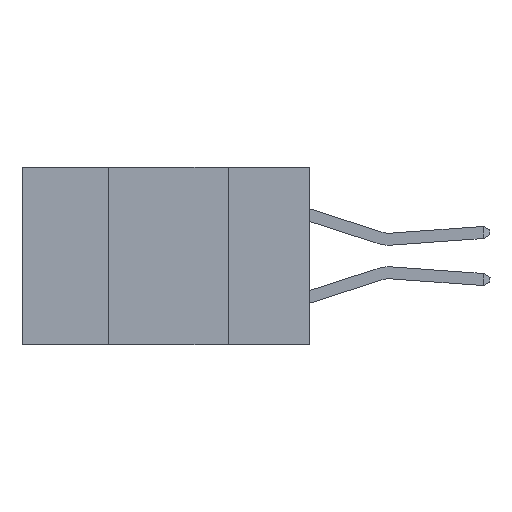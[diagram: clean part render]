
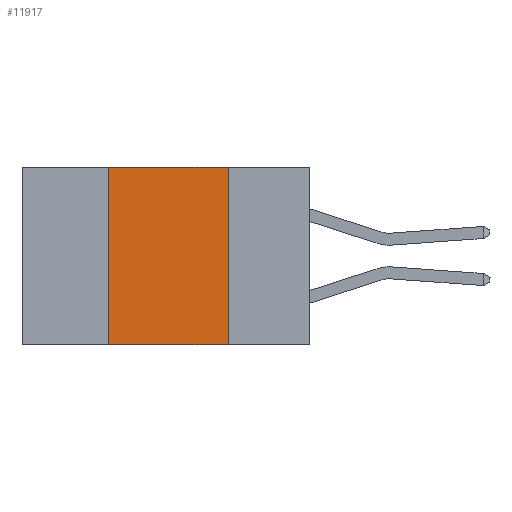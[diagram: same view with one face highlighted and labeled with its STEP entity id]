
A CAD part, left-side view. The second image highlights one B-rep face of the part: STEP entity #11917.
In plain terms, the highlighted planar face has unit normal (-1, 0, 0).
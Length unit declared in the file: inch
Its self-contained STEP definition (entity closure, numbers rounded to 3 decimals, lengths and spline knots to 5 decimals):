
#153 = FACE_OUTER_BOUND ( 'NONE', #10729, .T. ) ;
#1185 = ORIENTED_EDGE ( 'NONE', *, *, #19954, .F. ) ;
#1909 = DIRECTION ( 'NONE',  ( 1., 0., 0. ) ) ;
#2059 = VECTOR ( 'NONE', #17074, 39.37008 ) ;
#2104 = VERTEX_POINT ( 'NONE', #7624 ) ;
#2248 = CARTESIAN_POINT ( 'NONE',  ( 0., 0.17, -0.37 ) ) ;
#2817 = CARTESIAN_POINT ( 'NONE',  ( 0., 0.42, 0. ) ) ;
#3074 = LINE ( 'NONE', #8497, #19302 ) ;
#3381 = DIRECTION ( 'NONE',  ( 0., -1., 0. ) ) ;
#4059 = VERTEX_POINT ( 'NONE', #2248 ) ;
#5503 = ORIENTED_EDGE ( 'NONE', *, *, #12636, .F. ) ;
#6038 = DIRECTION ( 'NONE',  ( 0., 0., -1. ) ) ;
#6523 = LINE ( 'NONE', #17033, #9708 ) ;
#6775 = VECTOR ( 'NONE', #6038, 39.37008 ) ;
#7624 = CARTESIAN_POINT ( 'NONE',  ( 0., 0.42, 0. ) ) ;
#7852 = EDGE_CURVE ( 'NONE', #13060, #2104, #19563, .T. ) ;
#8497 = CARTESIAN_POINT ( 'NONE',  ( 0., 0.6, -0.37 ) ) ;
#8956 = ORIENTED_EDGE ( 'NONE', *, *, #7852, .F. ) ;
#9198 = DIRECTION ( 'NONE',  ( 0., -1., 0. ) ) ;
#9708 = VECTOR ( 'NONE', #9198, 39.37008 ) ;
#10729 = EDGE_LOOP ( 'NONE', ( #1185, #5503, #8956, #10933 ) ) ;
#10933 = ORIENTED_EDGE ( 'NONE', *, *, #15348, .T. ) ;
#11465 = PLANE ( 'NONE',  #15675 ) ;
#11917 = ADVANCED_FACE ( 'NONE', ( #153 ), #11465, .F. ) ;
#12118 = VERTEX_POINT ( 'NONE', #16066 ) ;
#12636 = EDGE_CURVE ( 'NONE', #2104, #12118, #6523, .T. ) ;
#12656 = CARTESIAN_POINT ( 'NONE',  ( 0., 0.42, -0.37 ) ) ;
#13060 = VERTEX_POINT ( 'NONE', #12656 ) ;
#13913 = CARTESIAN_POINT ( 'NONE',  ( 0., 0.17, 0. ) ) ;
#15348 = EDGE_CURVE ( 'NONE', #13060, #4059, #3074, .T. ) ;
#15675 = AXIS2_PLACEMENT_3D ( 'NONE', #16087, #1909, #17945 ) ;
#16066 = CARTESIAN_POINT ( 'NONE',  ( 0., 0.17, 0. ) ) ;
#16087 = CARTESIAN_POINT ( 'NONE',  ( 0., 0.6, 0. ) ) ;
#17033 = CARTESIAN_POINT ( 'NONE',  ( 0., 0.6, 0. ) ) ;
#17074 = DIRECTION ( 'NONE',  ( 0., 0., 1. ) ) ;
#17887 = LINE ( 'NONE', #13913, #6775 ) ;
#17945 = DIRECTION ( 'NONE',  ( 0., 0., -1. ) ) ;
#19302 = VECTOR ( 'NONE', #3381, 39.37008 ) ;
#19563 = LINE ( 'NONE', #2817, #2059 ) ;
#19954 = EDGE_CURVE ( 'NONE', #12118, #4059, #17887, .T. ) ;
